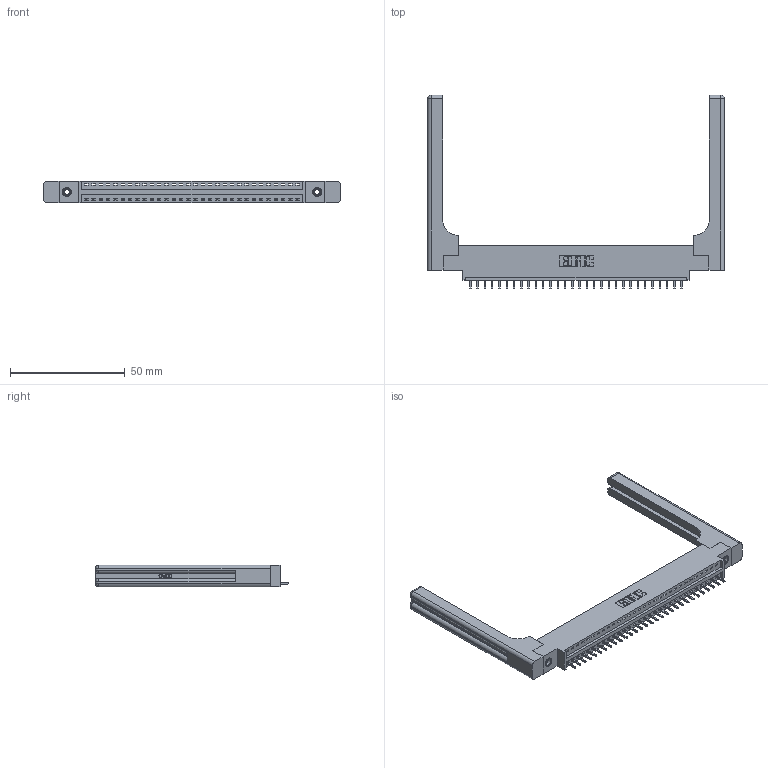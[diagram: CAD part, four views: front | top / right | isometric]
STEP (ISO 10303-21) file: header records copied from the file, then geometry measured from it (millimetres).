
FILE_DESCRIPTION (( 'STEP AP203' ), '1' );
FILE_NAME ('346-030-521-658.STEP', '2022-05-06T15:30:17', ( '' ), ( '' ), 'SwSTEP 2.0', 'SolidWorks 2020', '' );
FILE_SCHEMA (( 'CONFIG_CONTROL_DESIGN' ));
Length unit declared in the file: inch
Products named in the file (5): 345-250-001_345-250-001-102; 346-220-058_345-220-058; 346-030-521-658; 345-292-001_345-293-121; 346 Part_0.170 Offset - 0.156 Dia-TH
Assembly tree (35 placements, depth 2):
  346-030-521-658
    346 Part_0.170 Offset - 0.156 Dia-TH
    345-292-001_345-293-121  x30
    345-250-001_345-250-001-102  x2
    346-220-058_345-220-058  x2
Bounding box: 129.31 x 84.33 x 9.4 mm (x, y, z)
Volume: 19555.6 mm3; surface area: 19938.1 mm2
Topology: 35 solids, 35 shells, 2136 faces, 6323 edges, 4154 vertices
Faces by surface type: plane 1442, cylinder 634, bspline 36, cone 12, sphere 8, torus 4
Entity records: 25982 total; most frequent: CARTESIAN_POINT 5441, ORIENTED_EDGE 4200, DIRECTION 3744, EDGE_CURVE 2100, VECTOR 1756, LINE 1756, VERTEX_POINT 1390, AXIS2_PLACEMENT_3D 994
